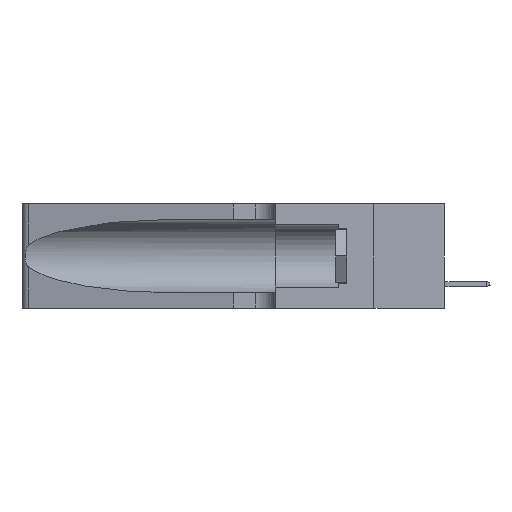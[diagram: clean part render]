
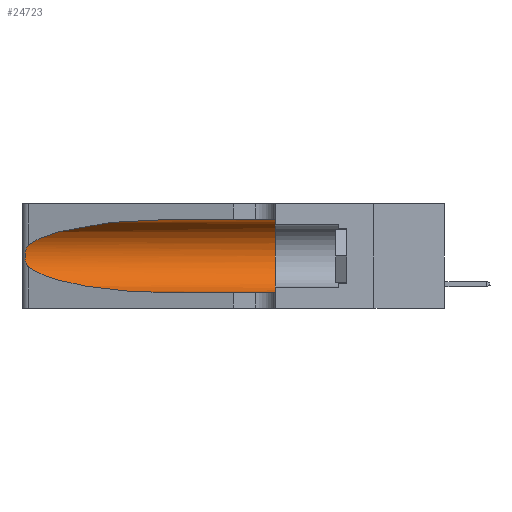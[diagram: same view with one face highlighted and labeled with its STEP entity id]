
A CAD part, left-side view. The second image highlights one B-rep face of the part: STEP entity #24723.
In plain terms, the highlighted cylindrical face has radius 3.308 mm (diameter 6.617 mm), a partial arc.
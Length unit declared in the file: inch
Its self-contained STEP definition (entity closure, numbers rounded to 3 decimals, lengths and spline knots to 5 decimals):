
#202 = VERTEX_POINT ( 'NONE', #2095 ) ;
#449 = CARTESIAN_POINT ( 'NONE',  ( 0.1305, 0.35, 0.05475 ) ) ;
#797 =( BOUNDED_CURVE ( )  B_SPLINE_CURVE ( 3, ( #32676, #8949, #40116, #3439 ),
 .UNSPECIFIED., .F., .F. ) 
 B_SPLINE_CURVE_WITH_KNOTS ( ( 4, 4 ),
 ( 3.44316, 4.71239 ),
 .UNSPECIFIED. ) 
 CURVE ( )  GEOMETRIC_REPRESENTATION_ITEM ( )  RATIONAL_B_SPLINE_CURVE ( ( 1., 0.87, 0.87, 1. ) ) 
 REPRESENTATION_ITEM ( '' )  );
#1034 = CARTESIAN_POINT ( 'NONE',  ( 0.26018, 1.23835, 0.19895 ) ) ;
#1503 = CARTESIAN_POINT ( 'NONE',  ( 0.25555, 1.22993, 0.14849 ) ) ;
#2095 = CARTESIAN_POINT ( 'NONE',  ( 0.25487, 1.22718, 0.14631 ) ) ;
#2423 = CARTESIAN_POINT ( 'NONE',  ( 0.1305, 1.61858, 0.31525 ) ) ;
#2805 = EDGE_LOOP ( 'NONE', ( #14686, #5503, #8518, #13938, #16724, #14104 ) ) ;
#3439 = CARTESIAN_POINT ( 'NONE',  ( 0.1305, 0.72297, 0.05475 ) ) ;
#3817 = VERTEX_POINT ( 'NONE', #19072 ) ;
#4179 = CARTESIAN_POINT ( 'NONE',  ( 0.25854, 1.2359, 0.20912 ) ) ;
#4486 = CARTESIAN_POINT ( 'NONE',  ( 0.26017, 1.23833, 0.17102 ) ) ;
#4701 = CARTESIAN_POINT ( 'NONE',  ( 0.1305, 1.61858, 0.05475 ) ) ;
#5488 = EDGE_CURVE ( 'NONE', #26737, #35274, #16135, .T. ) ;
#5503 = ORIENTED_EDGE ( 'NONE', *, *, #8840, .T. ) ;
#5751 = CARTESIAN_POINT ( 'NONE',  ( 0.1305, 0.35, 0.185 ) ) ;
#5888 = CARTESIAN_POINT ( 'NONE',  ( 0.1305, 0.72297, 0.31525 ) ) ;
#8518 = ORIENTED_EDGE ( 'NONE', *, *, #12239, .T. ) ;
#8610 = DIRECTION ( 'NONE',  ( 0., -1., 0. ) ) ;
#8840 = EDGE_CURVE ( 'NONE', #41167, #202, #11617, .T. ) ;
#8949 = CARTESIAN_POINT ( 'NONE',  ( 0.2373, 1.15595, 0.08982 ) ) ;
#9253 =( BOUNDED_CURVE ( )  B_SPLINE_CURVE ( 3, ( #5888, #41145, #9702, #29527 ),
 .UNSPECIFIED., .F., .T. ) 
 B_SPLINE_CURVE_WITH_KNOTS ( ( 4, 4 ),
 ( 1.5708, 2.84003 ),
 .UNSPECIFIED. ) 
 CURVE ( )  GEOMETRIC_REPRESENTATION_ITEM ( )  RATIONAL_B_SPLINE_CURVE ( ( 1., 0.87, 0.87, 1. ) ) 
 REPRESENTATION_ITEM ( '' )  );
#9437 = VECTOR ( 'NONE', #31293, 39.37008 ) ;
#9702 = CARTESIAN_POINT ( 'NONE',  ( 0.2373, 1.15595, 0.28018 ) ) ;
#9821 = DIRECTION ( 'NONE',  ( 0., 0., -1. ) ) ;
#10115 = AXIS2_PLACEMENT_3D ( 'NONE', #5751, #12159, #41616 ) ;
#10698 = CYLINDRICAL_SURFACE ( 'NONE', #19798, 0.13025 ) ;
#11080 = CARTESIAN_POINT ( 'NONE',  ( 0.25639, 1.23184, 0.21858 ) ) ;
#11211 = DIRECTION ( 'NONE',  ( 0., -1., 0. ) ) ;
#11617 = B_SPLINE_CURVE_WITH_KNOTS ( 'NONE', 3,
 ( #17877, #31093, #11080, #24185, #4179, #1034, #14074, #37077, #4486, #27627, #14531, #30952, #1503, #14679 ),
 .UNSPECIFIED., .F., .F.,
 ( 4, 2, 2, 2, 2, 2, 4 ),
 ( 0., 0.00027, 0.00053, 0.00107, 0.0016, 0.00187, 0.00214 ),
 .UNSPECIFIED. ) ;
#12159 = DIRECTION ( 'NONE',  ( 0., 1., 0. ) ) ;
#12239 = EDGE_CURVE ( 'NONE', #202, #26737, #797, .T. ) ;
#13938 = ORIENTED_EDGE ( 'NONE', *, *, #5488, .T. ) ;
#14074 = CARTESIAN_POINT ( 'NONE',  ( 0.26075, 1.23896, 0.19203 ) ) ;
#14104 = ORIENTED_EDGE ( 'NONE', *, *, #22918, .F. ) ;
#14531 = CARTESIAN_POINT ( 'NONE',  ( 0.25789, 1.23486, 0.15765 ) ) ;
#14679 = CARTESIAN_POINT ( 'NONE',  ( 0.25487, 1.22718, 0.14631 ) ) ;
#14686 = ORIENTED_EDGE ( 'NONE', *, *, #15501, .T. ) ;
#14819 = CARTESIAN_POINT ( 'NONE',  ( 0.1305, 0.35, 0.31525 ) ) ;
#15501 = EDGE_CURVE ( 'NONE', #3817, #41167, #9253, .T. ) ;
#16081 = CIRCLE ( 'NONE', #10115, 0.13025 ) ;
#16135 = LINE ( 'NONE', #4701, #9437 ) ;
#16601 = LINE ( 'NONE', #2423, #30437 ) ;
#16724 = ORIENTED_EDGE ( 'NONE', *, *, #22889, .F. ) ;
#17877 = CARTESIAN_POINT ( 'NONE',  ( 0.25487, 1.22718, 0.22369 ) ) ;
#19072 = CARTESIAN_POINT ( 'NONE',  ( 0.1305, 0.72297, 0.31525 ) ) ;
#19798 = AXIS2_PLACEMENT_3D ( 'NONE', #32188, #11211, #9821 ) ;
#22889 = EDGE_CURVE ( 'NONE', #25853, #35274, #16081, .T. ) ;
#22918 = EDGE_CURVE ( 'NONE', #3817, #25853, #16601, .T. ) ;
#23316 = CARTESIAN_POINT ( 'NONE',  ( 0.25487, 1.22718, 0.22369 ) ) ;
#24185 = CARTESIAN_POINT ( 'NONE',  ( 0.25787, 1.23484, 0.2124 ) ) ;
#24723 = ADVANCED_FACE ( 'NONE', ( #38515 ), #10698, .F. ) ;
#25853 = VERTEX_POINT ( 'NONE', #14819 ) ;
#26737 = VERTEX_POINT ( 'NONE', #37515 ) ;
#27627 = CARTESIAN_POINT ( 'NONE',  ( 0.25856, 1.23593, 0.16098 ) ) ;
#29527 = CARTESIAN_POINT ( 'NONE',  ( 0.25487, 1.22718, 0.22369 ) ) ;
#30437 = VECTOR ( 'NONE', #8610, 39.37008 ) ;
#30952 = CARTESIAN_POINT ( 'NONE',  ( 0.25639, 1.23186, 0.15144 ) ) ;
#31093 = CARTESIAN_POINT ( 'NONE',  ( 0.25555, 1.22994, 0.2215 ) ) ;
#31293 = DIRECTION ( 'NONE',  ( 0., -1., 0. ) ) ;
#32188 = CARTESIAN_POINT ( 'NONE',  ( 0.1305, 1.61858, 0.185 ) ) ;
#32676 = CARTESIAN_POINT ( 'NONE',  ( 0.25487, 1.22718, 0.14631 ) ) ;
#35274 = VERTEX_POINT ( 'NONE', #449 ) ;
#37077 = CARTESIAN_POINT ( 'NONE',  ( 0.26075, 1.23896, 0.178 ) ) ;
#37515 = CARTESIAN_POINT ( 'NONE',  ( 0.1305, 0.72297, 0.05475 ) ) ;
#38515 = FACE_OUTER_BOUND ( 'NONE', #2805, .T. ) ;
#40116 = CARTESIAN_POINT ( 'NONE',  ( 0.18966, 0.96281, 0.05475 ) ) ;
#41145 = CARTESIAN_POINT ( 'NONE',  ( 0.18966, 0.96281, 0.31525 ) ) ;
#41167 = VERTEX_POINT ( 'NONE', #23316 ) ;
#41616 = DIRECTION ( 'NONE',  ( 0., 0., 1. ) ) ;
